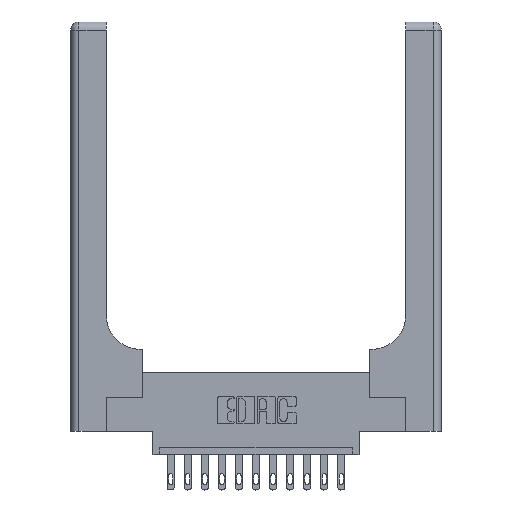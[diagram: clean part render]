
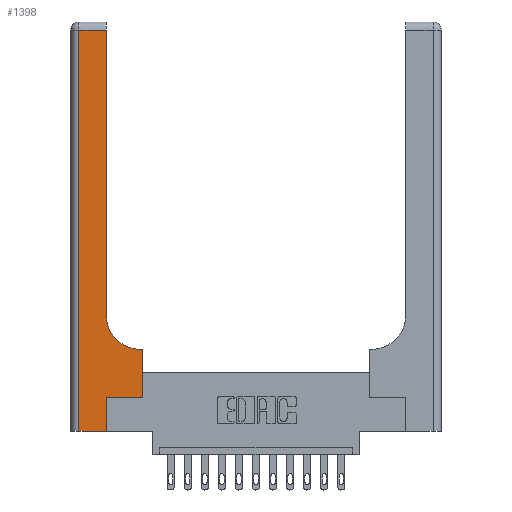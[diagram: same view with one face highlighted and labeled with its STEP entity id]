
A CAD part, top view. The second image highlights one B-rep face of the part: STEP entity #1398.
In plain terms, the highlighted planar face has unit normal (0, 0, 1).
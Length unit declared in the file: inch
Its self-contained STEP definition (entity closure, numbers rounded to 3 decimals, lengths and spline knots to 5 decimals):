
#87 = CARTESIAN_POINT ( 'NONE',  ( 0., 3., 0.37 ) ) ;
#446 = VECTOR ( 'NONE', #7905, 39.37008 ) ;
#563 = EDGE_CURVE ( 'NONE', #14550, #13988, #15461, .T. ) ;
#618 = CARTESIAN_POINT ( 'NONE',  ( 0.06, 3., 0.37 ) ) ;
#700 = DIRECTION ( 'NONE',  ( -1., 0., 0. ) ) ;
#1021 = VERTEX_POINT ( 'NONE', #5419 ) ;
#1398 = ADVANCED_FACE ( 'NONE', ( #11579 ), #10224, .F. ) ;
#1450 = DIRECTION ( 'NONE',  ( -1., 0., 0. ) ) ;
#1507 = VECTOR ( 'NONE', #4408, 39.37008 ) ;
#1626 = EDGE_CURVE ( 'NONE', #13988, #8942, #1944, .T. ) ;
#1944 = LINE ( 'NONE', #13767, #7001 ) ;
#2080 = CARTESIAN_POINT ( 'NONE',  ( 0.26, 0.85, 0.37 ) ) ;
#2495 = EDGE_CURVE ( 'NONE', #16368, #5220, #5841, .T. ) ;
#2501 = VECTOR ( 'NONE', #700, 39.37008 ) ;
#2856 = EDGE_CURVE ( 'NONE', #1021, #14003, #9606, .T. ) ;
#3076 = VECTOR ( 'NONE', #11911, 39.37008 ) ;
#3200 = DIRECTION ( 'NONE',  ( 0., 1., 0. ) ) ;
#3852 = CARTESIAN_POINT ( 'NONE',  ( 0., 2.94, 0.37 ) ) ;
#4006 = VECTOR ( 'NONE', #13045, 39.37008 ) ;
#4362 = CARTESIAN_POINT ( 'NONE',  ( 0.528, 0.25, 0.37 ) ) ;
#4397 = EDGE_CURVE ( 'NONE', #5656, #4802, #10589, .T. ) ;
#4408 = DIRECTION ( 'NONE',  ( 0., -1., 0. ) ) ;
#4775 = VECTOR ( 'NONE', #6980, 39.37008 ) ;
#4802 = VERTEX_POINT ( 'NONE', #14056 ) ;
#5005 = CARTESIAN_POINT ( 'NONE',  ( 0.51, 0.6, 0.37 ) ) ;
#5220 = VERTEX_POINT ( 'NONE', #11315 ) ;
#5358 = DIRECTION ( 'NONE',  ( 1., 0., 0. ) ) ;
#5394 = LINE ( 'NONE', #15773, #3076 ) ;
#5419 = CARTESIAN_POINT ( 'NONE',  ( 0.528, 0.25, 0.37 ) ) ;
#5484 = EDGE_LOOP ( 'NONE', ( #12598, #14427, #8280, #11533, #14457, #13685, #5803, #6883, #12580 ) ) ;
#5656 = VERTEX_POINT ( 'NONE', #12730 ) ;
#5803 = ORIENTED_EDGE ( 'NONE', *, *, #2856, .T. ) ;
#5841 = LINE ( 'NONE', #618, #1507 ) ;
#6817 = LINE ( 'NONE', #8519, #9160 ) ;
#6883 = ORIENTED_EDGE ( 'NONE', *, *, #10721, .T. ) ;
#6980 = DIRECTION ( 'NONE',  ( 0., 1., 0. ) ) ;
#7001 = VECTOR ( 'NONE', #3200, 39.37008 ) ;
#7318 = EDGE_CURVE ( 'NONE', #5220, #5656, #6817, .T. ) ;
#7905 = DIRECTION ( 'NONE',  ( -1., 0., 0. ) ) ;
#8280 = ORIENTED_EDGE ( 'NONE', *, *, #2495, .T. ) ;
#8519 = CARTESIAN_POINT ( 'NONE',  ( 0., 0., 0.37 ) ) ;
#8942 = VERTEX_POINT ( 'NONE', #12034 ) ;
#9160 = VECTOR ( 'NONE', #16349, 39.37008 ) ;
#9606 = LINE ( 'NONE', #4362, #4775 ) ;
#10224 = PLANE ( 'NONE',  #15347 ) ;
#10352 = AXIS2_PLACEMENT_3D ( 'NONE', #10587, #10426, #5358 ) ;
#10426 = DIRECTION ( 'NONE',  ( 0., 0., -1. ) ) ;
#10587 = CARTESIAN_POINT ( 'NONE',  ( 0.51, 0.85, 0.37 ) ) ;
#10589 = LINE ( 'NONE', #12890, #4006 ) ;
#10721 = EDGE_CURVE ( 'NONE', #14003, #14550, #10988, .T. ) ;
#10988 = LINE ( 'NONE', #13269, #2501 ) ;
#11049 = CARTESIAN_POINT ( 'NONE',  ( 0.06, 2.94, 0.37 ) ) ;
#11315 = CARTESIAN_POINT ( 'NONE',  ( 0.06, 0., 0.37 ) ) ;
#11533 = ORIENTED_EDGE ( 'NONE', *, *, #7318, .T. ) ;
#11579 = FACE_OUTER_BOUND ( 'NONE', #5484, .T. ) ;
#11911 = DIRECTION ( 'NONE',  ( 1., 0., 0. ) ) ;
#12034 = CARTESIAN_POINT ( 'NONE',  ( 0.26, 2.94, 0.37 ) ) ;
#12286 = EDGE_CURVE ( 'NONE', #4802, #1021, #5394, .T. ) ;
#12580 = ORIENTED_EDGE ( 'NONE', *, *, #563, .T. ) ;
#12598 = ORIENTED_EDGE ( 'NONE', *, *, #1626, .T. ) ;
#12730 = CARTESIAN_POINT ( 'NONE',  ( 0.265, 0., 0.37 ) ) ;
#12890 = CARTESIAN_POINT ( 'NONE',  ( 0.265, 0., 0.37 ) ) ;
#12977 = LINE ( 'NONE', #3852, #446 ) ;
#13045 = DIRECTION ( 'NONE',  ( 0., 1., 0. ) ) ;
#13269 = CARTESIAN_POINT ( 'NONE',  ( 0.26, 0.6, 0.37 ) ) ;
#13685 = ORIENTED_EDGE ( 'NONE', *, *, #12286, .T. ) ;
#13767 = CARTESIAN_POINT ( 'NONE',  ( 0.26, 3., 0.37 ) ) ;
#13988 = VERTEX_POINT ( 'NONE', #2080 ) ;
#14003 = VERTEX_POINT ( 'NONE', #15986 ) ;
#14056 = CARTESIAN_POINT ( 'NONE',  ( 0.265, 0.25, 0.37 ) ) ;
#14427 = ORIENTED_EDGE ( 'NONE', *, *, #16652, .T. ) ;
#14457 = ORIENTED_EDGE ( 'NONE', *, *, #4397, .T. ) ;
#14550 = VERTEX_POINT ( 'NONE', #5005 ) ;
#15347 = AXIS2_PLACEMENT_3D ( 'NONE', #87, #15362, #1450 ) ;
#15362 = DIRECTION ( 'NONE',  ( 0., 0., -1. ) ) ;
#15461 = CIRCLE ( 'NONE', #10352, 0.25 ) ;
#15773 = CARTESIAN_POINT ( 'NONE',  ( 0.265, 0.25, 0.37 ) ) ;
#15986 = CARTESIAN_POINT ( 'NONE',  ( 0.528, 0.6, 0.37 ) ) ;
#16349 = DIRECTION ( 'NONE',  ( 1., 0., 0. ) ) ;
#16368 = VERTEX_POINT ( 'NONE', #11049 ) ;
#16652 = EDGE_CURVE ( 'NONE', #8942, #16368, #12977, .T. ) ;
